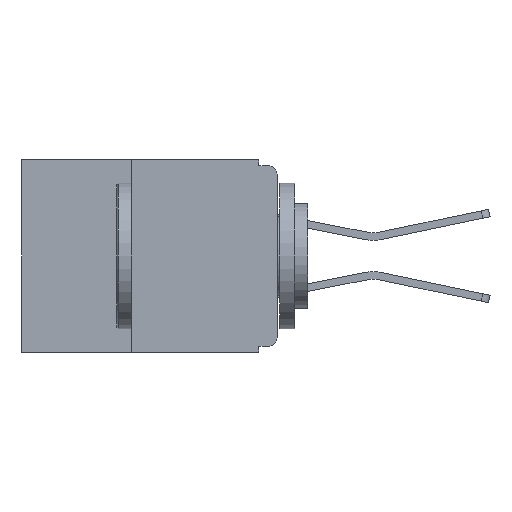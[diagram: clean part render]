
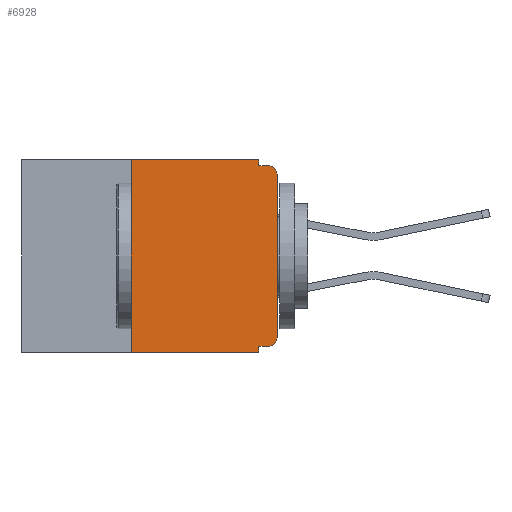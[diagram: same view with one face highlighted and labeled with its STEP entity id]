
A CAD part, left-side view. The second image highlights one B-rep face of the part: STEP entity #6928.
In plain terms, the highlighted planar face has unit normal (-1, 0, 0).
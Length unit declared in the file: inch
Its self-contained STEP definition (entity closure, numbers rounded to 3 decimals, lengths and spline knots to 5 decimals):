
#10 = EDGE_CURVE ( 'NONE', #5643, #11577, #15718, .T. ) ;
#73 = EDGE_CURVE ( 'NONE', #13049, #12463, #9389, .T. ) ;
#224 = PLANE ( 'NONE',  #6350 ) ;
#299 = DIRECTION ( 'NONE',  ( 0., 1., 0. ) ) ;
#686 = DIRECTION ( 'NONE',  ( 0., -1., 0. ) ) ;
#763 = ORIENTED_EDGE ( 'NONE', *, *, #6493, .T. ) ;
#1129 = LINE ( 'NONE', #2217, #4125 ) ;
#1593 = VECTOR ( 'NONE', #4313, 39.37008 ) ;
#1797 = ORIENTED_EDGE ( 'NONE', *, *, #4350, .T. ) ;
#2169 = VECTOR ( 'NONE', #2471, 39.37008 ) ;
#2217 = CARTESIAN_POINT ( 'NONE',  ( 0., 0.031, -0.33 ) ) ;
#2310 = EDGE_CURVE ( 'NONE', #7873, #13049, #8728, .T. ) ;
#2451 = CARTESIAN_POINT ( 'NONE',  ( 0., 0.437, 0. ) ) ;
#2471 = DIRECTION ( 'NONE',  ( 0., -1., 0. ) ) ;
#2881 = CARTESIAN_POINT ( 'NONE',  ( 0., 0.031, -0.33 ) ) ;
#3303 = VERTEX_POINT ( 'NONE', #13001 ) ;
#3782 = VERTEX_POINT ( 'NONE', #14405 ) ;
#4087 = VECTOR ( 'NONE', #686, 39.37008 ) ;
#4125 = VECTOR ( 'NONE', #4729, 39.37008 ) ;
#4313 = DIRECTION ( 'NONE',  ( 0., -1., 0. ) ) ;
#4350 = EDGE_CURVE ( 'NONE', #5643, #3782, #11846, .T. ) ;
#4464 = CARTESIAN_POINT ( 'NONE',  ( 0., 0., -0.01 ) ) ;
#4729 = DIRECTION ( 'NONE',  ( 0., 0., -1. ) ) ;
#5146 = CARTESIAN_POINT ( 'NONE',  ( 0., 0.015, -0.01 ) ) ;
#5643 = VERTEX_POINT ( 'NONE', #7404 ) ;
#5797 = EDGE_LOOP ( 'NONE', ( #16114, #9246, #7565, #15262, #11722, #14140, #763, #8775, #12173, #1797 ) ) ;
#5972 = VECTOR ( 'NONE', #299, 39.37008 ) ;
#6174 = DIRECTION ( 'NONE',  ( 0., 0., 1. ) ) ;
#6240 = DIRECTION ( 'NONE',  ( 0., 0., 1. ) ) ;
#6350 = AXIS2_PLACEMENT_3D ( 'NONE', #15725, #15398, #15601 ) ;
#6493 = EDGE_CURVE ( 'NONE', #7873, #8319, #7482, .T. ) ;
#6561 = EDGE_CURVE ( 'NONE', #14647, #6786, #9713, .T. ) ;
#6786 = VERTEX_POINT ( 'NONE', #5146 ) ;
#6928 = ADVANCED_FACE ( 'NONE', ( #7465 ), #224, .F. ) ;
#7218 = DIRECTION ( 'NONE',  ( 0., 0., -1. ) ) ;
#7241 = CARTESIAN_POINT ( 'NONE',  ( 0., 0.031, 0. ) ) ;
#7338 = CARTESIAN_POINT ( 'NONE',  ( 0., 0.437, -0.33 ) ) ;
#7404 = CARTESIAN_POINT ( 'NONE',  ( 0., 0.015, -0.32 ) ) ;
#7465 = FACE_OUTER_BOUND ( 'NONE', #5797, .T. ) ;
#7482 = LINE ( 'NONE', #7338, #4087 ) ;
#7565 = ORIENTED_EDGE ( 'NONE', *, *, #9969, .F. ) ;
#7566 = AXIS2_PLACEMENT_3D ( 'NONE', #11618, #11602, #11564 ) ;
#7612 = VECTOR ( 'NONE', #7218, 39.37008 ) ;
#7640 = CARTESIAN_POINT ( 'NONE',  ( 0., 0., -0.32 ) ) ;
#7873 = VERTEX_POINT ( 'NONE', #13746 ) ;
#8032 = LINE ( 'NONE', #7241, #7612 ) ;
#8319 = VERTEX_POINT ( 'NONE', #2881 ) ;
#8728 = LINE ( 'NONE', #10120, #14680 ) ;
#8775 = ORIENTED_EDGE ( 'NONE', *, *, #15778, .F. ) ;
#8915 = CARTESIAN_POINT ( 'NONE',  ( 0., 0., -0.025 ) ) ;
#9246 = ORIENTED_EDGE ( 'NONE', *, *, #6561, .T. ) ;
#9389 = LINE ( 'NONE', #2451, #2169 ) ;
#9613 = EDGE_CURVE ( 'NONE', #12463, #3303, #8032, .T. ) ;
#9619 = LINE ( 'NONE', #4464, #1593 ) ;
#9713 = CIRCLE ( 'NONE', #15506, 0.015 ) ;
#9969 = EDGE_CURVE ( 'NONE', #3303, #6786, #9619, .T. ) ;
#10120 = CARTESIAN_POINT ( 'NONE',  ( 0., 0.25, -0.33 ) ) ;
#10133 = VECTOR ( 'NONE', #6240, 39.37008 ) ;
#10470 = CARTESIAN_POINT ( 'NONE',  ( 0., 0.031, -0.32 ) ) ;
#11564 = DIRECTION ( 'NONE',  ( 0., 0., -1. ) ) ;
#11577 = VERTEX_POINT ( 'NONE', #10470 ) ;
#11602 = DIRECTION ( 'NONE',  ( -1., 0., 0. ) ) ;
#11618 = CARTESIAN_POINT ( 'NONE',  ( 0., 0.015, -0.305 ) ) ;
#11722 = ORIENTED_EDGE ( 'NONE', *, *, #73, .F. ) ;
#11846 = CIRCLE ( 'NONE', #7566, 0.015 ) ;
#12144 = CARTESIAN_POINT ( 'NONE',  ( 0., 0.25, 0. ) ) ;
#12173 = ORIENTED_EDGE ( 'NONE', *, *, #10, .F. ) ;
#12463 = VERTEX_POINT ( 'NONE', #13504 ) ;
#13001 = CARTESIAN_POINT ( 'NONE',  ( 0., 0.031, -0.01 ) ) ;
#13049 = VERTEX_POINT ( 'NONE', #12144 ) ;
#13504 = CARTESIAN_POINT ( 'NONE',  ( 0., 0.031, 0. ) ) ;
#13746 = CARTESIAN_POINT ( 'NONE',  ( 0., 0.25, -0.33 ) ) ;
#13890 = CARTESIAN_POINT ( 'NONE',  ( 0., 0., 0. ) ) ;
#14140 = ORIENTED_EDGE ( 'NONE', *, *, #2310, .F. ) ;
#14405 = CARTESIAN_POINT ( 'NONE',  ( 0., 0., -0.305 ) ) ;
#14647 = VERTEX_POINT ( 'NONE', #8915 ) ;
#14680 = VECTOR ( 'NONE', #6174, 39.37008 ) ;
#15262 = ORIENTED_EDGE ( 'NONE', *, *, #9613, .F. ) ;
#15398 = DIRECTION ( 'NONE',  ( 1., 0., 0. ) ) ;
#15506 = AXIS2_PLACEMENT_3D ( 'NONE', #16212, #16171, #16122 ) ;
#15601 = DIRECTION ( 'NONE',  ( 0., 0., -1. ) ) ;
#15718 = LINE ( 'NONE', #7640, #5972 ) ;
#15725 = CARTESIAN_POINT ( 'NONE',  ( 0., 0.437, 0. ) ) ;
#15778 = EDGE_CURVE ( 'NONE', #11577, #8319, #1129, .T. ) ;
#15851 = EDGE_CURVE ( 'NONE', #3782, #14647, #16457, .T. ) ;
#16114 = ORIENTED_EDGE ( 'NONE', *, *, #15851, .T. ) ;
#16122 = DIRECTION ( 'NONE',  ( 0., 0., -1. ) ) ;
#16171 = DIRECTION ( 'NONE',  ( -1., 0., 0. ) ) ;
#16212 = CARTESIAN_POINT ( 'NONE',  ( 0., 0.015, -0.025 ) ) ;
#16457 = LINE ( 'NONE', #13890, #10133 ) ;
